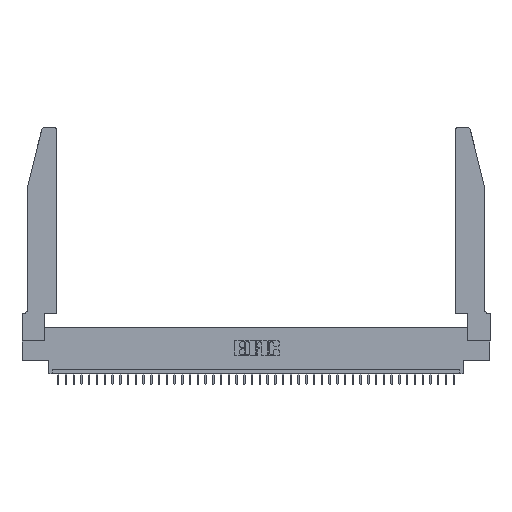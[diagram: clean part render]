
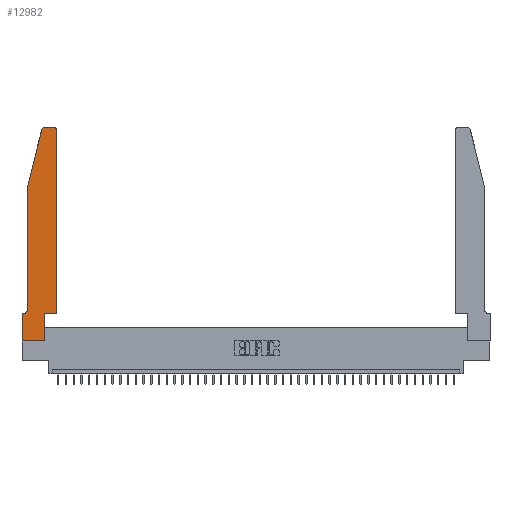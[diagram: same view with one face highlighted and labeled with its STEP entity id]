
A CAD part, top view. The second image highlights one B-rep face of the part: STEP entity #12982.
In plain terms, the highlighted planar face has unit normal (0, 0, 1).
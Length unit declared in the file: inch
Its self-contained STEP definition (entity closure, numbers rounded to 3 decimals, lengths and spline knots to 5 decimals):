
#323 = VERTEX_POINT ( 'NONE', #8353 ) ;
#509 = DIRECTION ( 'NONE',  ( 1., 0., 0. ) ) ;
#663 = LINE ( 'NONE', #13828, #4737 ) ;
#869 = EDGE_CURVE ( 'NONE', #3365, #25181, #42697, .T. ) ;
#1434 = LINE ( 'NONE', #18051, #28000 ) ;
#1572 = VERTEX_POINT ( 'NONE', #22884 ) ;
#1817 = CIRCLE ( 'NONE', #39795, 0.07 ) ;
#1840 = DIRECTION ( 'NONE',  ( 0., 0., 1. ) ) ;
#1951 = CARTESIAN_POINT ( 'NONE',  ( 0.4505, 2.72, 0.37 ) ) ;
#2159 = LINE ( 'NONE', #31599, #16784 ) ;
#2626 = EDGE_CURVE ( 'NONE', #10783, #1572, #1817, .T. ) ;
#2710 = ORIENTED_EDGE ( 'NONE', *, *, #39586, .T. ) ;
#3122 = DIRECTION ( 'NONE',  ( 0., 0., 1. ) ) ;
#3149 = ORIENTED_EDGE ( 'NONE', *, *, #37505, .T. ) ;
#3361 = VECTOR ( 'NONE', #34869, 39.37008 ) ;
#3365 = VERTEX_POINT ( 'NONE', #28733 ) ;
#4352 = CARTESIAN_POINT ( 'NONE',  ( 0.2605, 2.75, 0.37 ) ) ;
#4737 = VECTOR ( 'NONE', #40264, 39.37008 ) ;
#5304 = VECTOR ( 'NONE', #27399, 39.37008 ) ;
#5715 = CARTESIAN_POINT ( 'NONE',  ( 0.4205, 2.72, 0.37 ) ) ;
#5925 = DIRECTION ( 'NONE',  ( 0., -1., 0. ) ) ;
#6347 = PLANE ( 'NONE',  #18125 ) ;
#6932 = ORIENTED_EDGE ( 'NONE', *, *, #20882, .T. ) ;
#7056 = CARTESIAN_POINT ( 'NONE',  ( 0.0755, 0.35, 0.37 ) ) ;
#7271 = CARTESIAN_POINT ( 'NONE',  ( 0., 0., 0.37 ) ) ;
#7528 = CARTESIAN_POINT ( 'NONE',  ( 0.2865, 0.35, 0.37 ) ) ;
#8353 = CARTESIAN_POINT ( 'NONE',  ( 0.4205, 2.75, 0.37 ) ) ;
#8770 = CIRCLE ( 'NONE', #34404, 0.03 ) ;
#9162 = CARTESIAN_POINT ( 'NONE',  ( 0., 0., 0.37 ) ) ;
#9203 = EDGE_CURVE ( 'NONE', #323, #32853, #10805, .T. ) ;
#10783 = VERTEX_POINT ( 'NONE', #40651 ) ;
#10805 = LINE ( 'NONE', #4352, #31095 ) ;
#11145 = CARTESIAN_POINT ( 'NONE',  ( 0.0755, 2., 0.37 ) ) ;
#11815 = CIRCLE ( 'NONE', #21505, 0.03 ) ;
#12982 = ADVANCED_FACE ( 'NONE', ( #23869 ), #6347, .T. ) ;
#13311 = CARTESIAN_POINT ( 'NONE',  ( 0.25487, 2.72718, 0.37 ) ) ;
#13518 = CARTESIAN_POINT ( 'NONE',  ( 0.284, 2.72, 0.37 ) ) ;
#13828 = CARTESIAN_POINT ( 'NONE',  ( 0.0755, 2., 0.37 ) ) ;
#13888 = VERTEX_POINT ( 'NONE', #7528 ) ;
#14173 = DIRECTION ( 'NONE',  ( 0., 0., 1. ) ) ;
#14237 = LINE ( 'NONE', #27454, #18142 ) ;
#14269 = EDGE_CURVE ( 'NONE', #1572, #3365, #17632, .T. ) ;
#14403 = EDGE_CURVE ( 'NONE', #32853, #23636, #8770, .T. ) ;
#14699 = CARTESIAN_POINT ( 'NONE',  ( 0.0055, 0.42, 0.37 ) ) ;
#14889 = DIRECTION ( 'NONE',  ( 0., 1., 0. ) ) ;
#15701 = VERTEX_POINT ( 'NONE', #11145 ) ;
#15759 = VECTOR ( 'NONE', #24466, 39.37008 ) ;
#16063 = CARTESIAN_POINT ( 'NONE',  ( 0.4505, 0.35, 0.37 ) ) ;
#16518 = ORIENTED_EDGE ( 'NONE', *, *, #869, .T. ) ;
#16784 = VECTOR ( 'NONE', #14889, 39.37008 ) ;
#17588 = EDGE_CURVE ( 'NONE', #15701, #10783, #35070, .T. ) ;
#17632 = LINE ( 'NONE', #7056, #5304 ) ;
#17635 = EDGE_CURVE ( 'NONE', #25181, #41622, #30769, .T. ) ;
#17727 = CARTESIAN_POINT ( 'NONE',  ( 0., 0., 0.37 ) ) ;
#18038 = DIRECTION ( 'NONE',  ( 1., 0., 0. ) ) ;
#18051 = CARTESIAN_POINT ( 'NONE',  ( 0.2865, 0.35, 0.37 ) ) ;
#18125 = AXIS2_PLACEMENT_3D ( 'NONE', #30177, #3122, #509 ) ;
#18142 = VECTOR ( 'NONE', #24426, 39.37008 ) ;
#18433 = ORIENTED_EDGE ( 'NONE', *, *, #14269, .T. ) ;
#19695 = ORIENTED_EDGE ( 'NONE', *, *, #30237, .T. ) ;
#20882 = EDGE_CURVE ( 'NONE', #40659, #323, #11815, .T. ) ;
#21411 = DIRECTION ( 'NONE',  ( -1., 0., 0. ) ) ;
#21505 = AXIS2_PLACEMENT_3D ( 'NONE', #5715, #1840, #18038 ) ;
#22884 = CARTESIAN_POINT ( 'NONE',  ( 0.0055, 0.35, 0.37 ) ) ;
#23636 = VERTEX_POINT ( 'NONE', #13311 ) ;
#23869 = FACE_OUTER_BOUND ( 'NONE', #28691, .T. ) ;
#24243 = CARTESIAN_POINT ( 'NONE',  ( 0.0755, 2., 0.37 ) ) ;
#24426 = DIRECTION ( 'NONE',  ( 1., 0., 0. ) ) ;
#24466 = DIRECTION ( 'NONE',  ( 0., -1., 0. ) ) ;
#25181 = VERTEX_POINT ( 'NONE', #7271 ) ;
#25975 = VECTOR ( 'NONE', #5925, 39.37008 ) ;
#26636 = DIRECTION ( 'NONE',  ( -1., 0., 0. ) ) ;
#27074 = CARTESIAN_POINT ( 'NONE',  ( 0.2865, 0., 0.37 ) ) ;
#27399 = DIRECTION ( 'NONE',  ( -1., 0., 0. ) ) ;
#27454 = CARTESIAN_POINT ( 'NONE',  ( 0.4505, 0.35, 0.37 ) ) ;
#27886 = ORIENTED_EDGE ( 'NONE', *, *, #17635, .T. ) ;
#28000 = VECTOR ( 'NONE', #37575, 39.37008 ) ;
#28483 = ORIENTED_EDGE ( 'NONE', *, *, #35473, .T. ) ;
#28691 = EDGE_LOOP ( 'NONE', ( #36580, #42151, #19695, #30356, #33625, #18433, #16518, #27886, #2710, #28483, #3149, #6932 ) ) ;
#28733 = CARTESIAN_POINT ( 'NONE',  ( 0., 0.35, 0.37 ) ) ;
#30177 = CARTESIAN_POINT ( 'NONE',  ( 0., 0.35, 0.37 ) ) ;
#30237 = EDGE_CURVE ( 'NONE', #23636, #15701, #663, .T. ) ;
#30356 = ORIENTED_EDGE ( 'NONE', *, *, #17588, .T. ) ;
#30769 = LINE ( 'NONE', #17727, #3361 ) ;
#31095 = VECTOR ( 'NONE', #26636, 39.37008 ) ;
#31292 = CARTESIAN_POINT ( 'NONE',  ( 0.284, 2.75, 0.37 ) ) ;
#31599 = CARTESIAN_POINT ( 'NONE',  ( 0.4505, 0.35, 0.37 ) ) ;
#32853 = VERTEX_POINT ( 'NONE', #31292 ) ;
#33625 = ORIENTED_EDGE ( 'NONE', *, *, #2626, .T. ) ;
#34137 = DIRECTION ( 'NONE',  ( 1., 0., 0. ) ) ;
#34404 = AXIS2_PLACEMENT_3D ( 'NONE', #13518, #14173, #34137 ) ;
#34869 = DIRECTION ( 'NONE',  ( 1., 0., 0. ) ) ;
#35070 = LINE ( 'NONE', #24243, #15759 ) ;
#35287 = DIRECTION ( 'NONE',  ( 0., 0., -1. ) ) ;
#35473 = EDGE_CURVE ( 'NONE', #13888, #39870, #14237, .T. ) ;
#36580 = ORIENTED_EDGE ( 'NONE', *, *, #9203, .T. ) ;
#37505 = EDGE_CURVE ( 'NONE', #39870, #40659, #2159, .T. ) ;
#37575 = DIRECTION ( 'NONE',  ( 0., 1., 0. ) ) ;
#39586 = EDGE_CURVE ( 'NONE', #41622, #13888, #1434, .T. ) ;
#39795 = AXIS2_PLACEMENT_3D ( 'NONE', #14699, #35287, #21411 ) ;
#39870 = VERTEX_POINT ( 'NONE', #16063 ) ;
#40264 = DIRECTION ( 'NONE',  ( -0.239, -0.971, 0. ) ) ;
#40651 = CARTESIAN_POINT ( 'NONE',  ( 0.0755, 0.42, 0.37 ) ) ;
#40659 = VERTEX_POINT ( 'NONE', #1951 ) ;
#41622 = VERTEX_POINT ( 'NONE', #27074 ) ;
#42151 = ORIENTED_EDGE ( 'NONE', *, *, #14403, .T. ) ;
#42697 = LINE ( 'NONE', #9162, #25975 ) ;
